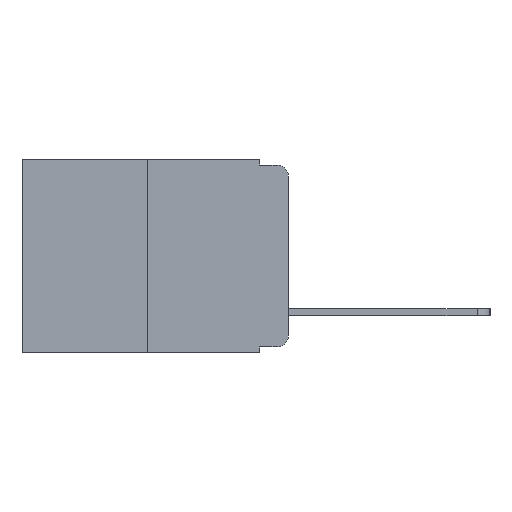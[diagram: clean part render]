
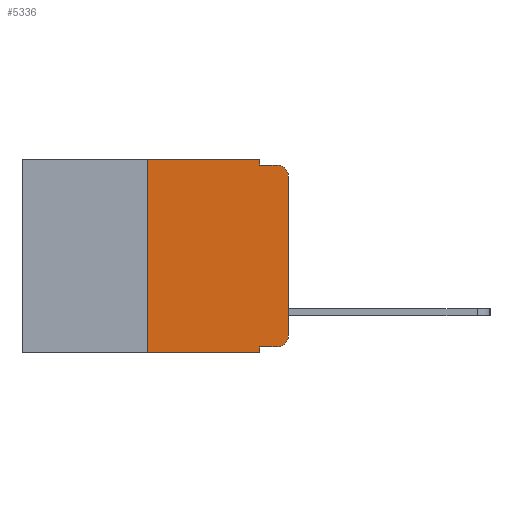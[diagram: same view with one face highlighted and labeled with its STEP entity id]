
A CAD part, left-side view. The second image highlights one B-rep face of the part: STEP entity #5336.
In plain terms, the highlighted planar face has unit normal (-1, 0, 0).
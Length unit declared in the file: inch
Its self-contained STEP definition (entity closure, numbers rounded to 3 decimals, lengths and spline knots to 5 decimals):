
#61 = VECTOR ( 'NONE', #2506, 39.37008 ) ;
#234 = LINE ( 'NONE', #11578, #2978 ) ;
#471 = CARTESIAN_POINT ( 'NONE',  ( 0., 0.051, 0. ) ) ;
#478 = LINE ( 'NONE', #10929, #8068 ) ;
#734 = ORIENTED_EDGE ( 'NONE', *, *, #7961, .F. ) ;
#1048 = DIRECTION ( 'NONE',  ( 0., 0., 1. ) ) ;
#1081 = ORIENTED_EDGE ( 'NONE', *, *, #8295, .F. ) ;
#1603 = CARTESIAN_POINT ( 'NONE',  ( 0., 0.25, 0. ) ) ;
#1762 = CARTESIAN_POINT ( 'NONE',  ( 0., 0.02, -0.03 ) ) ;
#1812 = EDGE_CURVE ( 'NONE', #7302, #2703, #478, .T. ) ;
#1900 = VERTEX_POINT ( 'NONE', #8664 ) ;
#1903 = VECTOR ( 'NONE', #8161, 39.37008 ) ;
#2013 = DIRECTION ( 'NONE',  ( 0., 0., -1. ) ) ;
#2064 = ORIENTED_EDGE ( 'NONE', *, *, #2721, .T. ) ;
#2280 = CIRCLE ( 'NONE', #8416, 0.02 ) ;
#2506 = DIRECTION ( 'NONE',  ( 0., -1., 0. ) ) ;
#2703 = VERTEX_POINT ( 'NONE', #4993 ) ;
#2721 = EDGE_CURVE ( 'NONE', #2703, #10230, #9683, .T. ) ;
#2749 = LINE ( 'NONE', #9303, #7412 ) ;
#2760 = DIRECTION ( 'NONE',  ( 0., 0., -1. ) ) ;
#2945 = DIRECTION ( 'NONE',  ( -1., 0., 0. ) ) ;
#2978 = VECTOR ( 'NONE', #1048, 39.37008 ) ;
#3022 = DIRECTION ( 'NONE',  ( 0., 0., -1. ) ) ;
#3465 = CARTESIAN_POINT ( 'NONE',  ( 0., 0.25, -0.343 ) ) ;
#3576 = EDGE_CURVE ( 'NONE', #10230, #4596, #234, .T. ) ;
#3655 = VERTEX_POINT ( 'NONE', #471 ) ;
#3803 = EDGE_CURVE ( 'NONE', #1900, #5397, #10064, .T. ) ;
#3857 = EDGE_CURVE ( 'NONE', #9134, #11011, #4443, .T. ) ;
#3880 = DIRECTION ( 'NONE',  ( 0., -1., 0. ) ) ;
#3982 = ORIENTED_EDGE ( 'NONE', *, *, #6426, .T. ) ;
#4246 = CARTESIAN_POINT ( 'NONE',  ( 0., 0.02, -0.313 ) ) ;
#4443 = LINE ( 'NONE', #1603, #1903 ) ;
#4520 = VECTOR ( 'NONE', #11054, 39.37008 ) ;
#4596 = VERTEX_POINT ( 'NONE', #10124 ) ;
#4993 = CARTESIAN_POINT ( 'NONE',  ( 0., 0.02, -0.333 ) ) ;
#5251 = VERTEX_POINT ( 'NONE', #9216 ) ;
#5303 = VECTOR ( 'NONE', #11182, 39.37008 ) ;
#5336 = ADVANCED_FACE ( 'NONE', ( #5734 ), #10183, .F. ) ;
#5397 = VERTEX_POINT ( 'NONE', #6802 ) ;
#5625 = ORIENTED_EDGE ( 'NONE', *, *, #3803, .F. ) ;
#5674 = CARTESIAN_POINT ( 'NONE',  ( 0., 0.25, 0. ) ) ;
#5734 = FACE_OUTER_BOUND ( 'NONE', #7971, .T. ) ;
#5784 = CARTESIAN_POINT ( 'NONE',  ( 0., 0.051, 0. ) ) ;
#6426 = EDGE_CURVE ( 'NONE', #9134, #5251, #2749, .T. ) ;
#6689 = EDGE_CURVE ( 'NONE', #4596, #5397, #2280, .T. ) ;
#6802 = CARTESIAN_POINT ( 'NONE',  ( 0., 0.02, -0.01 ) ) ;
#6934 = EDGE_CURVE ( 'NONE', #7302, #5251, #7706, .T. ) ;
#7302 = VERTEX_POINT ( 'NONE', #8998 ) ;
#7412 = VECTOR ( 'NONE', #3880, 39.37008 ) ;
#7600 = DIRECTION ( 'NONE',  ( 1., 0., 0. ) ) ;
#7706 = LINE ( 'NONE', #9405, #5303 ) ;
#7743 = ORIENTED_EDGE ( 'NONE', *, *, #3576, .T. ) ;
#7961 = EDGE_CURVE ( 'NONE', #3655, #1900, #9293, .T. ) ;
#7971 = EDGE_LOOP ( 'NONE', ( #7743, #10058, #5625, #734, #1081, #8547, #3982, #11132, #9086, #2064 ) ) ;
#8068 = VECTOR ( 'NONE', #11079, 39.37008 ) ;
#8161 = DIRECTION ( 'NONE',  ( 0., 0., 1. ) ) ;
#8274 = DIRECTION ( 'NONE',  ( -1., 0., 0. ) ) ;
#8295 = EDGE_CURVE ( 'NONE', #11011, #3655, #10651, .T. ) ;
#8357 = VECTOR ( 'NONE', #9724, 39.37008 ) ;
#8416 = AXIS2_PLACEMENT_3D ( 'NONE', #1762, #8274, #2760 ) ;
#8547 = ORIENTED_EDGE ( 'NONE', *, *, #3857, .F. ) ;
#8664 = CARTESIAN_POINT ( 'NONE',  ( 0., 0.051, -0.01 ) ) ;
#8998 = CARTESIAN_POINT ( 'NONE',  ( 0., 0.051, -0.333 ) ) ;
#9042 = AXIS2_PLACEMENT_3D ( 'NONE', #4246, #2945, #3022 ) ;
#9086 = ORIENTED_EDGE ( 'NONE', *, *, #1812, .T. ) ;
#9134 = VERTEX_POINT ( 'NONE', #3465 ) ;
#9216 = CARTESIAN_POINT ( 'NONE',  ( 0., 0.051, -0.343 ) ) ;
#9293 = LINE ( 'NONE', #5784, #4520 ) ;
#9303 = CARTESIAN_POINT ( 'NONE',  ( 0., 0.473, -0.343 ) ) ;
#9405 = CARTESIAN_POINT ( 'NONE',  ( 0., 0.051, 0. ) ) ;
#9683 = CIRCLE ( 'NONE', #9042, 0.02 ) ;
#9724 = DIRECTION ( 'NONE',  ( 0., -1., 0. ) ) ;
#9793 = CARTESIAN_POINT ( 'NONE',  ( 0., 0.051, -0.01 ) ) ;
#9908 = CARTESIAN_POINT ( 'NONE',  ( 0., 0., -0.313 ) ) ;
#10058 = ORIENTED_EDGE ( 'NONE', *, *, #6689, .T. ) ;
#10064 = LINE ( 'NONE', #9793, #61 ) ;
#10124 = CARTESIAN_POINT ( 'NONE',  ( 0., 0., -0.03 ) ) ;
#10183 = PLANE ( 'NONE',  #10392 ) ;
#10230 = VERTEX_POINT ( 'NONE', #9908 ) ;
#10392 = AXIS2_PLACEMENT_3D ( 'NONE', #11045, #7600, #2013 ) ;
#10651 = LINE ( 'NONE', #11400, #8357 ) ;
#10929 = CARTESIAN_POINT ( 'NONE',  ( 0., 0.051, -0.333 ) ) ;
#11011 = VERTEX_POINT ( 'NONE', #5674 ) ;
#11045 = CARTESIAN_POINT ( 'NONE',  ( 0., 0.473, 0. ) ) ;
#11054 = DIRECTION ( 'NONE',  ( 0., 0., -1. ) ) ;
#11079 = DIRECTION ( 'NONE',  ( 0., -1., 0. ) ) ;
#11132 = ORIENTED_EDGE ( 'NONE', *, *, #6934, .F. ) ;
#11182 = DIRECTION ( 'NONE',  ( 0., 0., -1. ) ) ;
#11400 = CARTESIAN_POINT ( 'NONE',  ( 0., 0.473, 0. ) ) ;
#11578 = CARTESIAN_POINT ( 'NONE',  ( 0., 0., 0. ) ) ;
